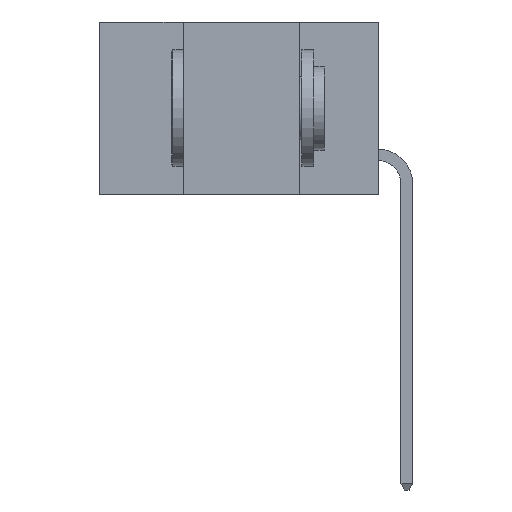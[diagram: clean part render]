
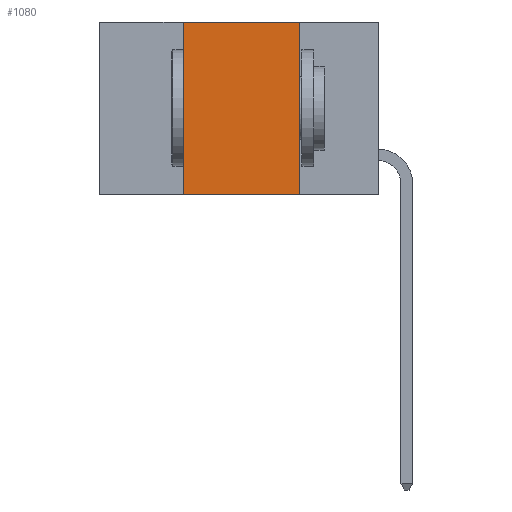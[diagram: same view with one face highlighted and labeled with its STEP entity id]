
A CAD part, left-side view. The second image highlights one B-rep face of the part: STEP entity #1080.
In plain terms, the highlighted planar face has unit normal (-1, 0, 0).
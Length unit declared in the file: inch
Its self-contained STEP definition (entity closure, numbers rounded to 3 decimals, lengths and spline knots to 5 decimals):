
#12 = VERTEX_POINT ( 'NONE', #3289 ) ;
#238 = PLANE ( 'NONE',  #17139 ) ;
#285 = CARTESIAN_POINT ( 'NONE',  ( 0., 0.6, 0. ) ) ;
#449 = VECTOR ( 'NONE', #8451, 39.37008 ) ;
#1080 = ADVANCED_FACE ( 'NONE', ( #10661 ), #238, .F. ) ;
#1616 = CARTESIAN_POINT ( 'NONE',  ( 0., 0.17, 0. ) ) ;
#1776 = LINE ( 'NONE', #2157, #8538 ) ;
#1779 = EDGE_LOOP ( 'NONE', ( #2030, #5688, #12694, #2452 ) ) ;
#1862 = VERTEX_POINT ( 'NONE', #17137 ) ;
#2030 = ORIENTED_EDGE ( 'NONE', *, *, #10623, .F. ) ;
#2157 = CARTESIAN_POINT ( 'NONE',  ( 0., 0.42, -0.37 ) ) ;
#2452 = ORIENTED_EDGE ( 'NONE', *, *, #9405, .T. ) ;
#3289 = CARTESIAN_POINT ( 'NONE',  ( 0., 0.42, -0.37 ) ) ;
#3325 = VECTOR ( 'NONE', #10899, 39.37008 ) ;
#4042 = VERTEX_POINT ( 'NONE', #1616 ) ;
#4175 = VECTOR ( 'NONE', #16421, 39.37008 ) ;
#4684 = LINE ( 'NONE', #14966, #449 ) ;
#5688 = ORIENTED_EDGE ( 'NONE', *, *, #6915, .F. ) ;
#5953 = CARTESIAN_POINT ( 'NONE',  ( 0., 0.17, -0.37 ) ) ;
#6885 = LINE ( 'NONE', #13436, #3325 ) ;
#6915 = EDGE_CURVE ( 'NONE', #1862, #4042, #4684, .T. ) ;
#8451 = DIRECTION ( 'NONE',  ( 0., -1., 0. ) ) ;
#8538 = VECTOR ( 'NONE', #8885, 39.37008 ) ;
#8885 = DIRECTION ( 'NONE',  ( 0., 0., 1. ) ) ;
#9405 = EDGE_CURVE ( 'NONE', #12, #13391, #6885, .T. ) ;
#10623 = EDGE_CURVE ( 'NONE', #4042, #13391, #14710, .T. ) ;
#10661 = FACE_OUTER_BOUND ( 'NONE', #1779, .T. ) ;
#10899 = DIRECTION ( 'NONE',  ( 0., -1., 0. ) ) ;
#11501 = EDGE_CURVE ( 'NONE', #12, #1862, #1776, .T. ) ;
#12694 = ORIENTED_EDGE ( 'NONE', *, *, #11501, .F. ) ;
#12733 = CARTESIAN_POINT ( 'NONE',  ( 0., 0.17, -0.37 ) ) ;
#13391 = VERTEX_POINT ( 'NONE', #12733 ) ;
#13436 = CARTESIAN_POINT ( 'NONE',  ( 0., 0.6, -0.37 ) ) ;
#14710 = LINE ( 'NONE', #5953, #4175 ) ;
#14966 = CARTESIAN_POINT ( 'NONE',  ( 0., 0.6, 0. ) ) ;
#16421 = DIRECTION ( 'NONE',  ( 0., 0., -1. ) ) ;
#17042 = DIRECTION ( 'NONE',  ( 1., 0., 0. ) ) ;
#17137 = CARTESIAN_POINT ( 'NONE',  ( 0., 0.42, 0. ) ) ;
#17139 = AXIS2_PLACEMENT_3D ( 'NONE', #285, #17042, #17323 ) ;
#17323 = DIRECTION ( 'NONE',  ( 0., 0., -1. ) ) ;
